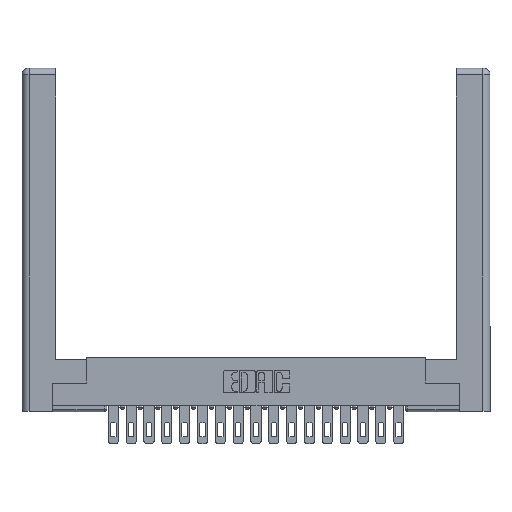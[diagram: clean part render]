
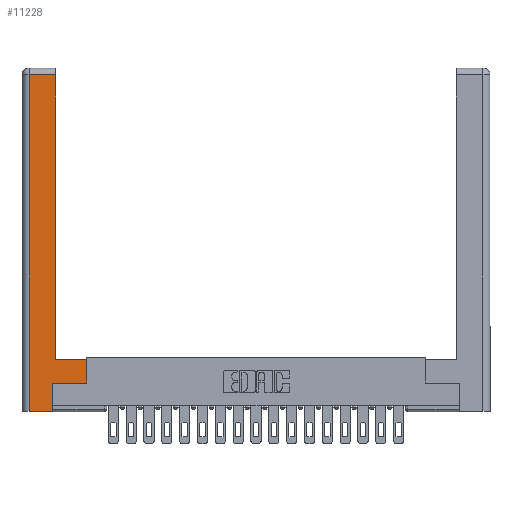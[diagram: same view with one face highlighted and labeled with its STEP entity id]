
A CAD part, top view. The second image highlights one B-rep face of the part: STEP entity #11228.
In plain terms, the highlighted planar face has unit normal (0, 0, 1).
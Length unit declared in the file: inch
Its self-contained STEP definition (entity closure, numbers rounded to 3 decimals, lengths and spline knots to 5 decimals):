
#596 = DIRECTION ( 'NONE',  ( 0., 0., -1. ) ) ;
#1108 = VECTOR ( 'NONE', #14921, 39.37008 ) ;
#1135 = CARTESIAN_POINT ( 'NONE',  ( 0.565, 0.45, 0. ) ) ;
#1516 = CARTESIAN_POINT ( 'NONE',  ( 0.565, 0.245, 0. ) ) ;
#1749 = DIRECTION ( 'NONE',  ( -1., 0., 0. ) ) ;
#1970 = LINE ( 'NONE', #1135, #13542 ) ;
#2038 = LINE ( 'NONE', #2343, #18640 ) ;
#2241 = CARTESIAN_POINT ( 'NONE',  ( 0.295, 0.45, 0. ) ) ;
#2257 = EDGE_CURVE ( 'NONE', #9697, #15354, #20132, .T. ) ;
#2293 = LINE ( 'NONE', #14713, #18900 ) ;
#2343 = CARTESIAN_POINT ( 'NONE',  ( 0.265, 0., 0. ) ) ;
#2829 = FACE_OUTER_BOUND ( 'NONE', #18238, .T. ) ;
#4272 = VECTOR ( 'NONE', #5854, 39.37008 ) ;
#4393 = LINE ( 'NONE', #2241, #1108 ) ;
#4475 = VECTOR ( 'NONE', #7349, 39.37008 ) ;
#5283 = VERTEX_POINT ( 'NONE', #13285 ) ;
#5854 = DIRECTION ( 'NONE',  ( 0., 1., 0. ) ) ;
#6145 = CARTESIAN_POINT ( 'NONE',  ( 0.295, 0.45, 0. ) ) ;
#6186 = ORIENTED_EDGE ( 'NONE', *, *, #18418, .T. ) ;
#7341 = CARTESIAN_POINT ( 'NONE',  ( 0.0615, 0., 0. ) ) ;
#7349 = DIRECTION ( 'NONE',  ( 0., 1., 0. ) ) ;
#7575 = ORIENTED_EDGE ( 'NONE', *, *, #8266, .T. ) ;
#8266 = EDGE_CURVE ( 'NONE', #10861, #14909, #11765, .T. ) ;
#9697 = VERTEX_POINT ( 'NONE', #6145 ) ;
#10136 = EDGE_CURVE ( 'NONE', #14507, #9697, #4393, .T. ) ;
#10719 = CARTESIAN_POINT ( 'NONE',  ( 0.0615, 0., 0. ) ) ;
#10861 = VERTEX_POINT ( 'NONE', #15364 ) ;
#11038 = VECTOR ( 'NONE', #15610, 39.37008 ) ;
#11228 = ADVANCED_FACE ( 'NONE', ( #2829 ), #16621, .F. ) ;
#11554 = VECTOR ( 'NONE', #13664, 39.37008 ) ;
#11765 = LINE ( 'NONE', #18483, #11038 ) ;
#11776 = EDGE_CURVE ( 'NONE', #15354, #15017, #2293, .T. ) ;
#11893 = CARTESIAN_POINT ( 'NONE',  ( 0.565, 0.45, 0. ) ) ;
#11995 = DIRECTION ( 'NONE',  ( 1., 0., 0. ) ) ;
#12266 = CARTESIAN_POINT ( 'NONE',  ( 0.265, 0.245, 0. ) ) ;
#12355 = CARTESIAN_POINT ( 'NONE',  ( 0.295, 2.94, 0. ) ) ;
#12504 = ORIENTED_EDGE ( 'NONE', *, *, #13892, .T. ) ;
#12518 = ORIENTED_EDGE ( 'NONE', *, *, #11776, .T. ) ;
#13032 = LINE ( 'NONE', #12266, #4475 ) ;
#13200 = EDGE_CURVE ( 'NONE', #15017, #15930, #16331, .T. ) ;
#13240 = DIRECTION ( 'NONE',  ( -1., 0., 0. ) ) ;
#13285 = CARTESIAN_POINT ( 'NONE',  ( 0.265, 0., 0. ) ) ;
#13356 = EDGE_CURVE ( 'NONE', #14909, #14507, #1970, .T. ) ;
#13542 = VECTOR ( 'NONE', #13801, 39.37008 ) ;
#13664 = DIRECTION ( 'NONE',  ( 0., -1., 0. ) ) ;
#13801 = DIRECTION ( 'NONE',  ( 0., 1., 0. ) ) ;
#13892 = EDGE_CURVE ( 'NONE', #5283, #10861, #13032, .T. ) ;
#14507 = VERTEX_POINT ( 'NONE', #11893 ) ;
#14713 = CARTESIAN_POINT ( 'NONE',  ( 0.0615, 2.94, 0. ) ) ;
#14909 = VERTEX_POINT ( 'NONE', #1516 ) ;
#14921 = DIRECTION ( 'NONE',  ( -1., 0., 0. ) ) ;
#15017 = VERTEX_POINT ( 'NONE', #19729 ) ;
#15165 = ORIENTED_EDGE ( 'NONE', *, *, #10136, .T. ) ;
#15354 = VERTEX_POINT ( 'NONE', #12355 ) ;
#15364 = CARTESIAN_POINT ( 'NONE',  ( 0.265, 0.245, 0. ) ) ;
#15476 = CARTESIAN_POINT ( 'NONE',  ( 0.295, 3., 0. ) ) ;
#15610 = DIRECTION ( 'NONE',  ( 1., 0., 0. ) ) ;
#15930 = VERTEX_POINT ( 'NONE', #10719 ) ;
#16331 = LINE ( 'NONE', #7341, #11554 ) ;
#16621 = PLANE ( 'NONE',  #20307 ) ;
#18238 = EDGE_LOOP ( 'NONE', ( #18557, #12518, #19287, #6186, #12504, #7575, #19054, #15165 ) ) ;
#18418 = EDGE_CURVE ( 'NONE', #15930, #5283, #2038, .T. ) ;
#18483 = CARTESIAN_POINT ( 'NONE',  ( 0.565, 0.245, 0. ) ) ;
#18557 = ORIENTED_EDGE ( 'NONE', *, *, #2257, .T. ) ;
#18640 = VECTOR ( 'NONE', #11995, 39.37008 ) ;
#18900 = VECTOR ( 'NONE', #1749, 39.37008 ) ;
#19054 = ORIENTED_EDGE ( 'NONE', *, *, #13356, .T. ) ;
#19287 = ORIENTED_EDGE ( 'NONE', *, *, #13200, .T. ) ;
#19729 = CARTESIAN_POINT ( 'NONE',  ( 0.0615, 2.94, 0. ) ) ;
#19842 = CARTESIAN_POINT ( 'NONE',  ( 0., 0., 0. ) ) ;
#20132 = LINE ( 'NONE', #15476, #4272 ) ;
#20307 = AXIS2_PLACEMENT_3D ( 'NONE', #19842, #596, #13240 ) ;
